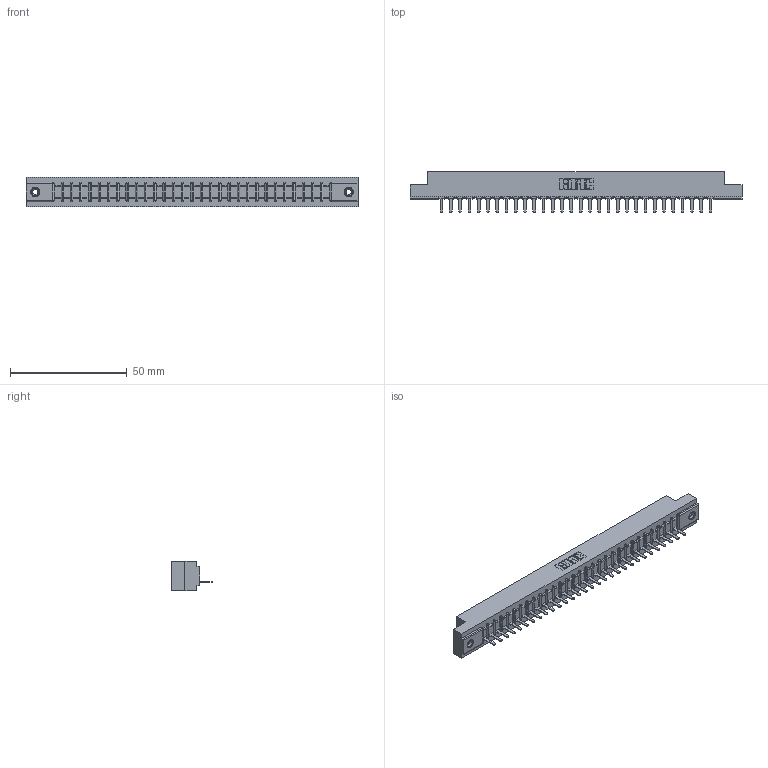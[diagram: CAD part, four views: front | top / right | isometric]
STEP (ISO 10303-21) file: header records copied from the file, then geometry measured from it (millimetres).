
FILE_DESCRIPTION (( 'STEP AP203' ), '1' );
FILE_NAME ('357-030-521-108.STEP', '2018-08-09T09:17:00', ( '' ), ( '' ), 'SwSTEP 2.0', 'SolidWorks 2016', '' );
FILE_SCHEMA (( 'CONFIG_CONTROL_DESIGN' ));
Length unit declared in the file: inch
Products named in the file (4): 357-030-521-108; 307 Part_.156 Dia Mounting Holes; 307-290-002_521; 345-250-001_345-250-003-102
Assembly tree (33 placements, depth 2):
  357-030-521-108
    307 Part_.156 Dia Mounting Holes
    307-290-002_521  x30
    345-250-001_345-250-003-102  x2
Bounding box: 141.88 x 17.42 x 12.7 mm (x, y, z)
Volume: 15089.2 mm3; surface area: 18734.5 mm2
Topology: 33 solids, 33 shells, 2429 faces, 7419 edges, 4854 vertices
Faces by surface type: plane 1452, cylinder 899, sphere 62, cone 12, torus 4
Entity records: 29101 total; most frequent: CARTESIAN_POINT 4887, ORIENTED_EDGE 4870, DIRECTION 4763, EDGE_CURVE 2435, LINE 1859, VECTOR 1859, VERTEX_POINT 1576, AXIS2_PLACEMENT_3D 1452
